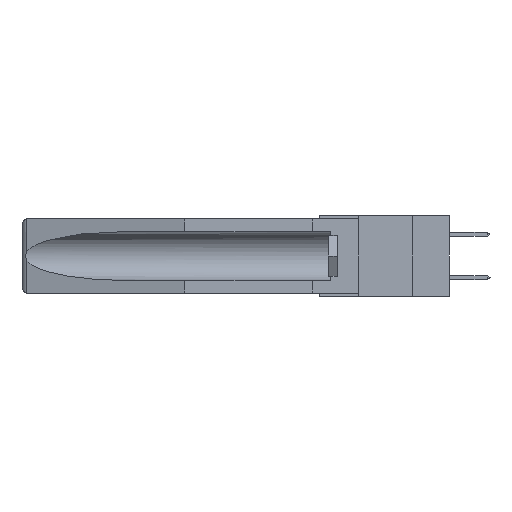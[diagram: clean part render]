
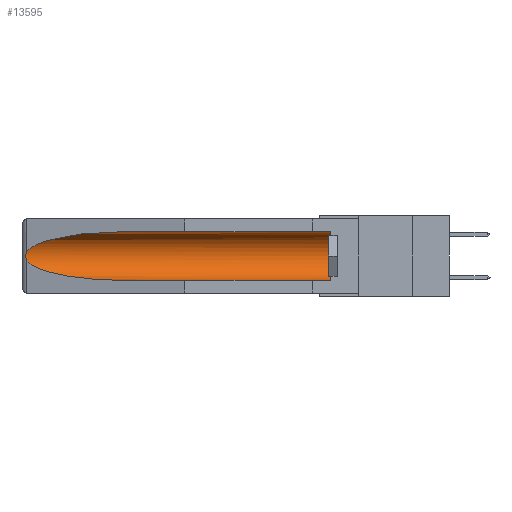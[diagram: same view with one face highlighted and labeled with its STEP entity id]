
A CAD part, left-side view. The second image highlights one B-rep face of the part: STEP entity #13595.
In plain terms, the highlighted cylindrical face has radius 2.857 mm (diameter 5.715 mm), a partial arc.
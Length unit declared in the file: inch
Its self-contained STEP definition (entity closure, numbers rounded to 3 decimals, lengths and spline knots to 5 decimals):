
#338 = CARTESIAN_POINT ( 'NONE',  ( 0.21114, 1.30732, -0.059 ) ) ;
#354 = CARTESIAN_POINT ( 'NONE',  ( 0.26537, 1.52718, -0.14972 ) ) ;
#521 = EDGE_CURVE ( 'NONE', #7361, #6675, #6724, .T. ) ;
#772 = DIRECTION ( 'NONE',  ( 0., 1., 0. ) ) ;
#1207 = CARTESIAN_POINT ( 'NONE',  ( 0.2675, 1.53308, -0.17534 ) ) ;
#1479 = AXIS2_PLACEMENT_3D ( 'NONE', #7071, #8636, #7204 ) ;
#1503 = VERTEX_POINT ( 'NONE', #354 ) ;
#1752 = DIRECTION ( 'NONE',  ( 0., -1., 0. ) ) ;
#2294 = AXIS2_PLACEMENT_3D ( 'NONE', #6013, #1752, #6203 ) ;
#3268 = ORIENTED_EDGE ( 'NONE', *, *, #6344, .F. ) ;
#3698 = CARTESIAN_POINT ( 'NONE',  ( 0.155, 1.07973, -0.284 ) ) ;
#3760 = CARTESIAN_POINT ( 'NONE',  ( 0.21114, 1.30732, -0.284 ) ) ;
#4183 = CARTESIAN_POINT ( 'NONE',  ( 0.155, 1.07973, -0.059 ) ) ;
#4410 = CARTESIAN_POINT ( 'NONE',  ( 0.155, -0.30754, -0.284 ) ) ;
#5307 = CARTESIAN_POINT ( 'NONE',  ( 0.155, -0.30754, -0.059 ) ) ;
#5635 = VERTEX_POINT ( 'NONE', #4183 ) ;
#5683 = CARTESIAN_POINT ( 'NONE',  ( 0.26537, 1.52718, -0.14972 ) ) ;
#5808 = CIRCLE ( 'NONE', #2294, 0.1125 ) ;
#6013 = CARTESIAN_POINT ( 'NONE',  ( 0.155, 0.126, -0.1715 ) ) ;
#6203 = DIRECTION ( 'NONE',  ( 0., 0., 1. ) ) ;
#6344 = EDGE_CURVE ( 'NONE', #13765, #6675, #10731, .T. ) ;
#6675 = VERTEX_POINT ( 'NONE', #13480 ) ;
#6724 =( BOUNDED_CURVE ( )  B_SPLINE_CURVE ( 3, ( #8084, #12630, #3760, #3698 ),
 .UNSPECIFIED., .F., .F. ) 
 B_SPLINE_CURVE_WITH_KNOTS ( ( 4, 4 ),
 ( 0.1948, 1.5708 ),
 .UNSPECIFIED. ) 
 CURVE ( )  GEOMETRIC_REPRESENTATION_ITEM ( )  RATIONAL_B_SPLINE_CURVE ( ( 1., 0.848, 0.848, 1. ) ) 
 REPRESENTATION_ITEM ( '' )  );
#6942 = CARTESIAN_POINT ( 'NONE',  ( 0.2673, 1.5327, -0.16383 ) ) ;
#7009 = CARTESIAN_POINT ( 'NONE',  ( 0.26597, 1.52961, -0.15275 ) ) ;
#7019 = LINE ( 'NONE', #5307, #14665 ) ;
#7071 = CARTESIAN_POINT ( 'NONE',  ( 0.155, -0.30754, -0.1715 ) ) ;
#7204 = DIRECTION ( 'NONE',  ( 0., 0., 1. ) ) ;
#7328 =( BOUNDED_CURVE ( )  B_SPLINE_CURVE ( 3, ( #16828, #338, #18130, #16563 ),
 .UNSPECIFIED., .F., .F. ) 
 B_SPLINE_CURVE_WITH_KNOTS ( ( 4, 4 ),
 ( 4.71239, 6.08839 ),
 .UNSPECIFIED. ) 
 CURVE ( )  GEOMETRIC_REPRESENTATION_ITEM ( )  RATIONAL_B_SPLINE_CURVE ( ( 1., 0.848, 0.848, 1. ) ) 
 REPRESENTATION_ITEM ( '' )  );
#7336 = EDGE_CURVE ( 'NONE', #13765, #8146, #5808, .T. ) ;
#7361 = VERTEX_POINT ( 'NONE', #17457 ) ;
#7919 = ORIENTED_EDGE ( 'NONE', *, *, #14473, .T. ) ;
#8084 = CARTESIAN_POINT ( 'NONE',  ( 0.26537, 1.52718, -0.19328 ) ) ;
#8124 = CARTESIAN_POINT ( 'NONE',  ( 0.2673, 1.53269, -0.17917 ) ) ;
#8146 = VERTEX_POINT ( 'NONE', #9812 ) ;
#8390 = FACE_OUTER_BOUND ( 'NONE', #15054, .T. ) ;
#8636 = DIRECTION ( 'NONE',  ( 0., 1., 0. ) ) ;
#8906 = EDGE_CURVE ( 'NONE', #1503, #7361, #11056, .T. ) ;
#9078 = DIRECTION ( 'NONE',  ( 0., 1., 0. ) ) ;
#9360 = CARTESIAN_POINT ( 'NONE',  ( 0.155, 0.126, -0.284 ) ) ;
#9730 = ORIENTED_EDGE ( 'NONE', *, *, #7336, .T. ) ;
#9812 = CARTESIAN_POINT ( 'NONE',  ( 0.155, 0.126, -0.059 ) ) ;
#10087 = CARTESIAN_POINT ( 'NONE',  ( 0.2675, 1.53308, -0.16763 ) ) ;
#10460 = ORIENTED_EDGE ( 'NONE', *, *, #12869, .T. ) ;
#10731 = LINE ( 'NONE', #4410, #18119 ) ;
#10738 = CYLINDRICAL_SURFACE ( 'NONE', #1479, 0.1125 ) ;
#11056 = B_SPLINE_CURVE_WITH_KNOTS ( 'NONE', 3,
 ( #5683, #7009, #15955, #6942, #10087, #1207, #8124, #14342, #14018, #17313 ),
 .UNSPECIFIED., .F., .F.,
 ( 4, 2, 2, 2, 4 ),
 ( 0., 0.00029, 0.00058, 0.00087, 0.00117 ),
 .UNSPECIFIED. ) ;
#12630 = CARTESIAN_POINT ( 'NONE',  ( 0.25451, 1.48313, -0.24835 ) ) ;
#12869 = EDGE_CURVE ( 'NONE', #8146, #5635, #7019, .T. ) ;
#13480 = CARTESIAN_POINT ( 'NONE',  ( 0.155, 1.07973, -0.284 ) ) ;
#13595 = ADVANCED_FACE ( 'NONE', ( #8390 ), #10738, .F. ) ;
#13765 = VERTEX_POINT ( 'NONE', #9360 ) ;
#14018 = CARTESIAN_POINT ( 'NONE',  ( 0.26597, 1.5296, -0.19026 ) ) ;
#14342 = CARTESIAN_POINT ( 'NONE',  ( 0.26655, 1.53094, -0.18657 ) ) ;
#14473 = EDGE_CURVE ( 'NONE', #5635, #1503, #7328, .T. ) ;
#14665 = VECTOR ( 'NONE', #772, 39.37008 ) ;
#15054 = EDGE_LOOP ( 'NONE', ( #7919, #15553, #18723, #3268, #9730, #10460 ) ) ;
#15553 = ORIENTED_EDGE ( 'NONE', *, *, #8906, .T. ) ;
#15955 = CARTESIAN_POINT ( 'NONE',  ( 0.26654, 1.53092, -0.15636 ) ) ;
#16563 = CARTESIAN_POINT ( 'NONE',  ( 0.26537, 1.52718, -0.14972 ) ) ;
#16828 = CARTESIAN_POINT ( 'NONE',  ( 0.155, 1.07973, -0.059 ) ) ;
#17313 = CARTESIAN_POINT ( 'NONE',  ( 0.26537, 1.52718, -0.19328 ) ) ;
#17457 = CARTESIAN_POINT ( 'NONE',  ( 0.26537, 1.52718, -0.19328 ) ) ;
#18119 = VECTOR ( 'NONE', #9078, 39.37008 ) ;
#18130 = CARTESIAN_POINT ( 'NONE',  ( 0.25451, 1.48313, -0.09465 ) ) ;
#18723 = ORIENTED_EDGE ( 'NONE', *, *, #521, .T. ) ;
